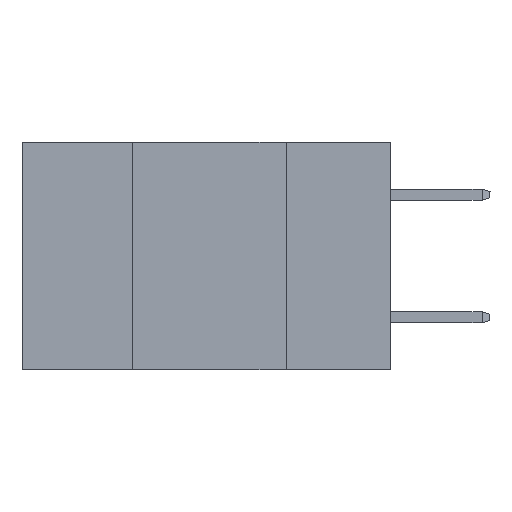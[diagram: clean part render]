
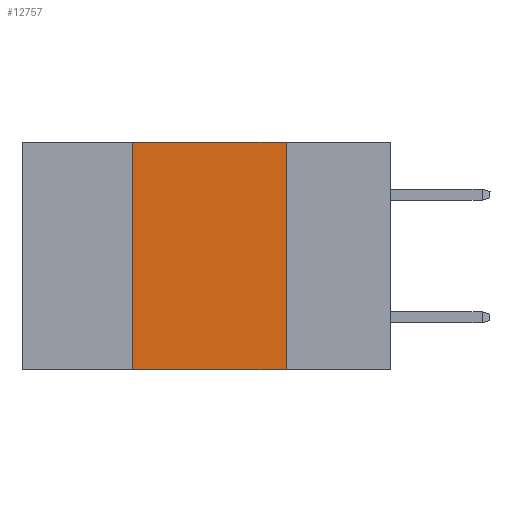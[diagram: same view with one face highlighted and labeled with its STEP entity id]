
A CAD part, left-side view. The second image highlights one B-rep face of the part: STEP entity #12757.
In plain terms, the highlighted planar face has unit normal (-1, 0, 0).
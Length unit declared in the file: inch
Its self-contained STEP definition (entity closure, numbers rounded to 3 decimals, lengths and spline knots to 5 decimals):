
#29 = EDGE_CURVE ( 'NONE', #16038, #19133, #17008, .T. ) ;
#209 = CARTESIAN_POINT ( 'NONE',  ( 0., 0.6, 0. ) ) ;
#1504 = DIRECTION ( 'NONE',  ( 0., -1., 0. ) ) ;
#1637 = EDGE_CURVE ( 'NONE', #7589, #14632, #9649, .T. ) ;
#2225 = LINE ( 'NONE', #2327, #4426 ) ;
#2327 = CARTESIAN_POINT ( 'NONE',  ( 0., 0.42, 0. ) ) ;
#3020 = DIRECTION ( 'NONE',  ( 1., 0., 0. ) ) ;
#3232 = CARTESIAN_POINT ( 'NONE',  ( 0., 0.6, -0.37 ) ) ;
#4202 = ORIENTED_EDGE ( 'NONE', *, *, #29, .F. ) ;
#4426 = VECTOR ( 'NONE', #11779, 39.37008 ) ;
#5306 = LINE ( 'NONE', #16802, #18961 ) ;
#6261 = ORIENTED_EDGE ( 'NONE', *, *, #16521, .F. ) ;
#7349 = ORIENTED_EDGE ( 'NONE', *, *, #1637, .T. ) ;
#7589 = VERTEX_POINT ( 'NONE', #8412 ) ;
#8412 = CARTESIAN_POINT ( 'NONE',  ( 0., 0.42, -0.37 ) ) ;
#9190 = CARTESIAN_POINT ( 'NONE',  ( 0., 0.17, -0.37 ) ) ;
#9335 = CARTESIAN_POINT ( 'NONE',  ( 0., 0.17, 0. ) ) ;
#9649 = LINE ( 'NONE', #3232, #14540 ) ;
#10568 = EDGE_CURVE ( 'NONE', #7589, #16038, #2225, .T. ) ;
#11200 = ORIENTED_EDGE ( 'NONE', *, *, #10568, .F. ) ;
#11384 = EDGE_LOOP ( 'NONE', ( #6261, #4202, #11200, #7349 ) ) ;
#11491 = PLANE ( 'NONE',  #19233 ) ;
#11779 = DIRECTION ( 'NONE',  ( 0., 0., 1. ) ) ;
#12477 = CARTESIAN_POINT ( 'NONE',  ( 0., 0.6, 0. ) ) ;
#12757 = ADVANCED_FACE ( 'NONE', ( #16903 ), #11491, .F. ) ;
#13121 = VECTOR ( 'NONE', #18719, 39.37008 ) ;
#14540 = VECTOR ( 'NONE', #1504, 39.37008 ) ;
#14632 = VERTEX_POINT ( 'NONE', #9190 ) ;
#14975 = DIRECTION ( 'NONE',  ( 0., 0., -1. ) ) ;
#16038 = VERTEX_POINT ( 'NONE', #17903 ) ;
#16453 = DIRECTION ( 'NONE',  ( 0., 0., -1. ) ) ;
#16521 = EDGE_CURVE ( 'NONE', #19133, #14632, #5306, .T. ) ;
#16802 = CARTESIAN_POINT ( 'NONE',  ( 0., 0.17, 0. ) ) ;
#16903 = FACE_OUTER_BOUND ( 'NONE', #11384, .T. ) ;
#17008 = LINE ( 'NONE', #12477, #13121 ) ;
#17903 = CARTESIAN_POINT ( 'NONE',  ( 0., 0.42, 0. ) ) ;
#18719 = DIRECTION ( 'NONE',  ( 0., -1., 0. ) ) ;
#18961 = VECTOR ( 'NONE', #14975, 39.37008 ) ;
#19133 = VERTEX_POINT ( 'NONE', #9335 ) ;
#19233 = AXIS2_PLACEMENT_3D ( 'NONE', #209, #3020, #16453 ) ;
